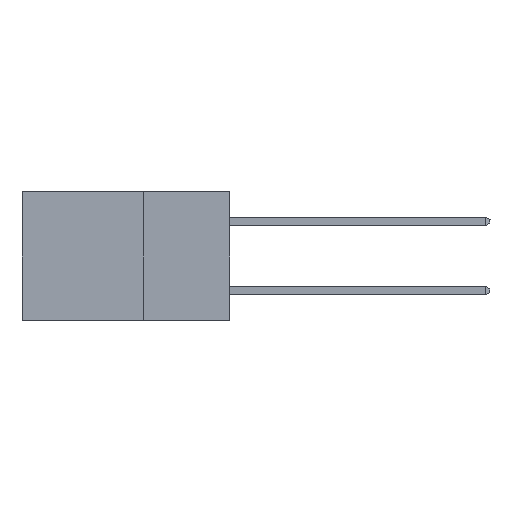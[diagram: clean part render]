
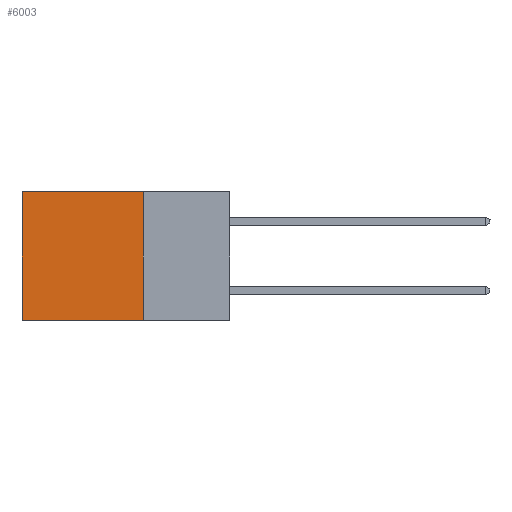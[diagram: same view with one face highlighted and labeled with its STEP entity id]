
A CAD part, left-side view. The second image highlights one B-rep face of the part: STEP entity #6003.
In plain terms, the highlighted planar face has unit normal (-1, 0, 0).
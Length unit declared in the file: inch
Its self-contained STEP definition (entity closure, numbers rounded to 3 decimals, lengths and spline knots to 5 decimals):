
#359 = DIRECTION ( 'NONE',  ( 0., 1., 0. ) ) ;
#569 = ORIENTED_EDGE ( 'NONE', *, *, #11832, .F. ) ;
#2466 = DIRECTION ( 'NONE',  ( 0., 0., -1. ) ) ;
#3383 = VERTEX_POINT ( 'NONE', #12465 ) ;
#3657 = DIRECTION ( 'NONE',  ( 0., 0., -1. ) ) ;
#3832 = LINE ( 'NONE', #18537, #9378 ) ;
#4614 = CARTESIAN_POINT ( 'NONE',  ( 0.2615, 0.25, -0.37 ) ) ;
#4984 = EDGE_CURVE ( 'NONE', #3383, #6020, #15617, .T. ) ;
#5441 = PLANE ( 'NONE',  #10046 ) ;
#6003 = ADVANCED_FACE ( 'NONE', ( #12413 ), #5441, .F. ) ;
#6020 = VERTEX_POINT ( 'NONE', #16339 ) ;
#7035 = VERTEX_POINT ( 'NONE', #13743 ) ;
#7078 = VECTOR ( 'NONE', #14962, 39.37008 ) ;
#7114 = DIRECTION ( 'NONE',  ( 0., 1., 0. ) ) ;
#7692 = LINE ( 'NONE', #19993, #7078 ) ;
#8508 = VERTEX_POINT ( 'NONE', #16750 ) ;
#9378 = VECTOR ( 'NONE', #359, 39.37008 ) ;
#10046 = AXIS2_PLACEMENT_3D ( 'NONE', #14535, #19567, #3657 ) ;
#10744 = ORIENTED_EDGE ( 'NONE', *, *, #22619, .T. ) ;
#11832 = EDGE_CURVE ( 'NONE', #6020, #7035, #3832, .T. ) ;
#12413 = FACE_OUTER_BOUND ( 'NONE', #18987, .T. ) ;
#12465 = CARTESIAN_POINT ( 'NONE',  ( 0.2615, 0.25, 0. ) ) ;
#13478 = VECTOR ( 'NONE', #2466, 39.37008 ) ;
#13743 = CARTESIAN_POINT ( 'NONE',  ( 0.2615, 0.6, -0.37 ) ) ;
#14535 = CARTESIAN_POINT ( 'NONE',  ( 0.2615, 0.25, -0.37 ) ) ;
#14962 = DIRECTION ( 'NONE',  ( 0., 0., -1. ) ) ;
#15617 = LINE ( 'NONE', #4614, #13478 ) ;
#16177 = LINE ( 'NONE', #23472, #20413 ) ;
#16339 = CARTESIAN_POINT ( 'NONE',  ( 0.2615, 0.25, -0.37 ) ) ;
#16750 = CARTESIAN_POINT ( 'NONE',  ( 0.2615, 0.6, 0. ) ) ;
#17328 = ORIENTED_EDGE ( 'NONE', *, *, #22500, .T. ) ;
#18537 = CARTESIAN_POINT ( 'NONE',  ( 0.2615, 0.25, -0.37 ) ) ;
#18987 = EDGE_LOOP ( 'NONE', ( #10744, #569, #21686, #17328 ) ) ;
#19567 = DIRECTION ( 'NONE',  ( 1., 0., 0. ) ) ;
#19993 = CARTESIAN_POINT ( 'NONE',  ( 0.2615, 0.6, -0.37 ) ) ;
#20413 = VECTOR ( 'NONE', #7114, 39.37008 ) ;
#21686 = ORIENTED_EDGE ( 'NONE', *, *, #4984, .F. ) ;
#22500 = EDGE_CURVE ( 'NONE', #3383, #8508, #16177, .T. ) ;
#22619 = EDGE_CURVE ( 'NONE', #8508, #7035, #7692, .T. ) ;
#23472 = CARTESIAN_POINT ( 'NONE',  ( 0.2615, 0.25, 0. ) ) ;
